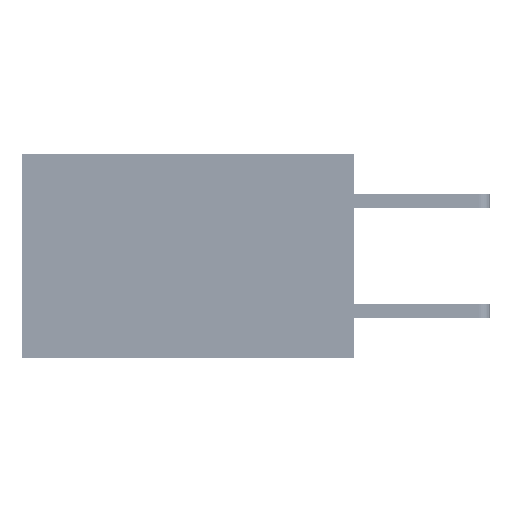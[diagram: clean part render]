
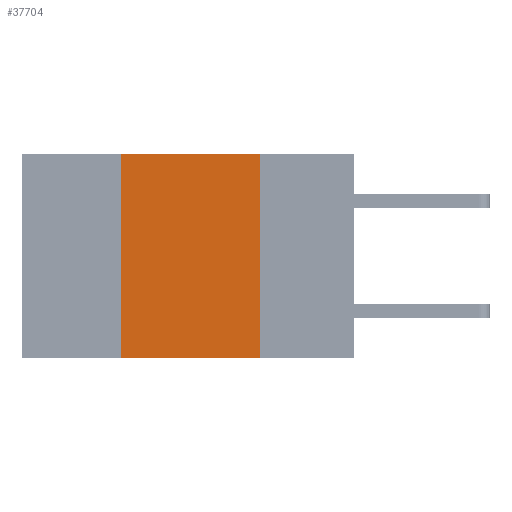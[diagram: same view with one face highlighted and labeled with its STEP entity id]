
A CAD part, left-side view. The second image highlights one B-rep face of the part: STEP entity #37704.
In plain terms, the highlighted planar face has unit normal (-1, 0, 0).
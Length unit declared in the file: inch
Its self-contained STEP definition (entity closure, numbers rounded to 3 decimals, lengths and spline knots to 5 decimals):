
#1201 = LINE ( 'NONE', #42997, #36377 ) ;
#1270 = VECTOR ( 'NONE', #5640, 39.37008 ) ;
#2522 = LINE ( 'NONE', #9668, #45907 ) ;
#3020 = LINE ( 'NONE', #39708, #1270 ) ;
#3106 = AXIS2_PLACEMENT_3D ( 'NONE', #17770, #43808, #47437 ) ;
#3548 = CARTESIAN_POINT ( 'NONE',  ( 0., 0.42, -0.37 ) ) ;
#5640 = DIRECTION ( 'NONE',  ( 0., -1., 0. ) ) ;
#6046 = EDGE_CURVE ( 'NONE', #39241, #7428, #3020, .T. ) ;
#7428 = VERTEX_POINT ( 'NONE', #21810 ) ;
#8309 = FACE_OUTER_BOUND ( 'NONE', #28263, .T. ) ;
#9668 = CARTESIAN_POINT ( 'NONE',  ( 0., 0.6, 0. ) ) ;
#11320 = LINE ( 'NONE', #37702, #15402 ) ;
#14478 = EDGE_CURVE ( 'NONE', #39241, #34977, #1201, .T. ) ;
#15311 = DIRECTION ( 'NONE',  ( 0., 0., -1. ) ) ;
#15402 = VECTOR ( 'NONE', #15311, 39.37008 ) ;
#17770 = CARTESIAN_POINT ( 'NONE',  ( 0., 0.6, 0. ) ) ;
#21100 = ORIENTED_EDGE ( 'NONE', *, *, #28814, .F. ) ;
#21810 = CARTESIAN_POINT ( 'NONE',  ( 0., 0.17, -0.37 ) ) ;
#23636 = VERTEX_POINT ( 'NONE', #41608 ) ;
#25010 = PLANE ( 'NONE',  #3106 ) ;
#28263 = EDGE_LOOP ( 'NONE', ( #21100, #47358, #42684, #47506 ) ) ;
#28814 = EDGE_CURVE ( 'NONE', #23636, #7428, #11320, .T. ) ;
#29322 = EDGE_CURVE ( 'NONE', #34977, #23636, #2522, .T. ) ;
#31853 = DIRECTION ( 'NONE',  ( 0., 0., 1. ) ) ;
#34977 = VERTEX_POINT ( 'NONE', #45418 ) ;
#36377 = VECTOR ( 'NONE', #31853, 39.37008 ) ;
#37702 = CARTESIAN_POINT ( 'NONE',  ( 0., 0.17, 0. ) ) ;
#37704 = ADVANCED_FACE ( 'NONE', ( #8309 ), #25010, .F. ) ;
#39241 = VERTEX_POINT ( 'NONE', #3548 ) ;
#39708 = CARTESIAN_POINT ( 'NONE',  ( 0., 0.6, -0.37 ) ) ;
#40424 = DIRECTION ( 'NONE',  ( 0., -1., 0. ) ) ;
#41608 = CARTESIAN_POINT ( 'NONE',  ( 0., 0.17, 0. ) ) ;
#42684 = ORIENTED_EDGE ( 'NONE', *, *, #14478, .F. ) ;
#42997 = CARTESIAN_POINT ( 'NONE',  ( 0., 0.42, 0. ) ) ;
#43808 = DIRECTION ( 'NONE',  ( 1., 0., 0. ) ) ;
#45418 = CARTESIAN_POINT ( 'NONE',  ( 0., 0.42, 0. ) ) ;
#45907 = VECTOR ( 'NONE', #40424, 39.37008 ) ;
#47358 = ORIENTED_EDGE ( 'NONE', *, *, #29322, .F. ) ;
#47437 = DIRECTION ( 'NONE',  ( 0., 0., -1. ) ) ;
#47506 = ORIENTED_EDGE ( 'NONE', *, *, #6046, .T. ) ;
